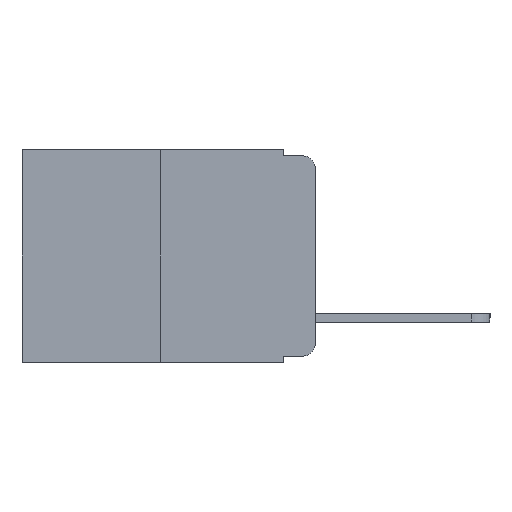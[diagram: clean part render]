
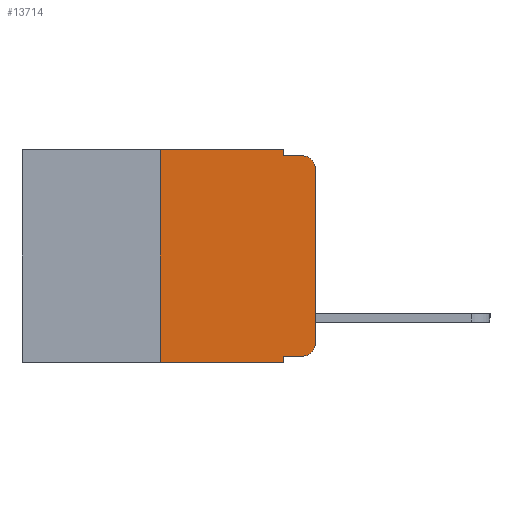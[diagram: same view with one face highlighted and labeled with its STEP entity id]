
A CAD part, left-side view. The second image highlights one B-rep face of the part: STEP entity #13714.
In plain terms, the highlighted planar face has unit normal (-1, 0, 0).
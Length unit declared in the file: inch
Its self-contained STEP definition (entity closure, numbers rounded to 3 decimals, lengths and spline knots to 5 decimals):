
#218 = VECTOR ( 'NONE', #4773, 39.37008 ) ;
#249 = AXIS2_PLACEMENT_3D ( 'NONE', #5105, #11500, #5154 ) ;
#748 = LINE ( 'NONE', #1525, #9641 ) ;
#808 = CARTESIAN_POINT ( 'NONE',  ( 0., 0.25, 0. ) ) ;
#854 = EDGE_CURVE ( 'NONE', #11794, #7351, #8269, .T. ) ;
#1036 = EDGE_CURVE ( 'NONE', #11684, #6754, #11219, .T. ) ;
#1085 = DIRECTION ( 'NONE',  ( -1., 0., 0. ) ) ;
#1188 = CARTESIAN_POINT ( 'NONE',  ( 0., 0.02, -0.333 ) ) ;
#1525 = CARTESIAN_POINT ( 'NONE',  ( 0., 0.473, 0. ) ) ;
#1909 = PLANE ( 'NONE',  #249 ) ;
#2154 = CIRCLE ( 'NONE', #10046, 0.02 ) ;
#2180 = ORIENTED_EDGE ( 'NONE', *, *, #4214, .F. ) ;
#2294 = CARTESIAN_POINT ( 'NONE',  ( 0., 0.051, -0.01 ) ) ;
#2528 = EDGE_CURVE ( 'NONE', #7351, #7688, #5343, .T. ) ;
#2683 = CARTESIAN_POINT ( 'NONE',  ( 0., 0., -0.313 ) ) ;
#3416 = CARTESIAN_POINT ( 'NONE',  ( 0., 0.051, -0.01 ) ) ;
#3449 = CARTESIAN_POINT ( 'NONE',  ( 0., 0.051, -0.343 ) ) ;
#3455 = EDGE_CURVE ( 'NONE', #4340, #9997, #6809, .T. ) ;
#3601 = CARTESIAN_POINT ( 'NONE',  ( 0., 0.02, -0.313 ) ) ;
#3839 = ORIENTED_EDGE ( 'NONE', *, *, #2528, .T. ) ;
#4214 = EDGE_CURVE ( 'NONE', #6754, #10799, #748, .T. ) ;
#4245 = EDGE_CURVE ( 'NONE', #11835, #6197, #5792, .T. ) ;
#4275 = VECTOR ( 'NONE', #12640, 39.37008 ) ;
#4340 = VERTEX_POINT ( 'NONE', #12952 ) ;
#4430 = DIRECTION ( 'NONE',  ( 0., -1., 0. ) ) ;
#4698 = ORIENTED_EDGE ( 'NONE', *, *, #5234, .F. ) ;
#4773 = DIRECTION ( 'NONE',  ( 0., 0., 1. ) ) ;
#4866 = ORIENTED_EDGE ( 'NONE', *, *, #9236, .T. ) ;
#5105 = CARTESIAN_POINT ( 'NONE',  ( 0., 0.473, 0. ) ) ;
#5154 = DIRECTION ( 'NONE',  ( 0., 0., -1. ) ) ;
#5234 = EDGE_CURVE ( 'NONE', #10799, #11835, #7107, .T. ) ;
#5343 = LINE ( 'NONE', #9181, #10650 ) ;
#5631 = VECTOR ( 'NONE', #13531, 39.37008 ) ;
#5707 = CARTESIAN_POINT ( 'NONE',  ( 0., 0.051, 0. ) ) ;
#5792 = LINE ( 'NONE', #2294, #11431 ) ;
#5940 = LINE ( 'NONE', #13579, #11244 ) ;
#6018 = ORIENTED_EDGE ( 'NONE', *, *, #6727, .T. ) ;
#6197 = VERTEX_POINT ( 'NONE', #6860 ) ;
#6575 = DIRECTION ( 'NONE',  ( 0., -1., 0. ) ) ;
#6727 = EDGE_CURVE ( 'NONE', #11684, #9997, #11610, .T. ) ;
#6754 = VERTEX_POINT ( 'NONE', #808 ) ;
#6809 = LINE ( 'NONE', #11252, #9307 ) ;
#6849 = DIRECTION ( 'NONE',  ( -1., 0., 0. ) ) ;
#6860 = CARTESIAN_POINT ( 'NONE',  ( 0., 0.02, -0.01 ) ) ;
#7107 = LINE ( 'NONE', #5707, #4275 ) ;
#7212 = DIRECTION ( 'NONE',  ( 0., 0., -1. ) ) ;
#7351 = VERTEX_POINT ( 'NONE', #2683 ) ;
#7504 = CARTESIAN_POINT ( 'NONE',  ( 0., 0.02, -0.03 ) ) ;
#7688 = VERTEX_POINT ( 'NONE', #13433 ) ;
#7718 = CARTESIAN_POINT ( 'NONE',  ( 0., 0.25, 0. ) ) ;
#8189 = DIRECTION ( 'NONE',  ( 0., 0., -1. ) ) ;
#8269 = CIRCLE ( 'NONE', #8898, 0.02 ) ;
#8362 = DIRECTION ( 'NONE',  ( 0., -1., 0. ) ) ;
#8593 = DIRECTION ( 'NONE',  ( 0., 0., -1. ) ) ;
#8898 = AXIS2_PLACEMENT_3D ( 'NONE', #3601, #6849, #7212 ) ;
#9177 = DIRECTION ( 'NONE',  ( 0., 0., 1. ) ) ;
#9181 = CARTESIAN_POINT ( 'NONE',  ( 0., 0., 0. ) ) ;
#9236 = EDGE_CURVE ( 'NONE', #7688, #6197, #2154, .T. ) ;
#9241 = EDGE_LOOP ( 'NONE', ( #3839, #4866, #11827, #4698, #2180, #11332, #6018, #9847, #13621, #12162 ) ) ;
#9307 = VECTOR ( 'NONE', #8189, 39.37008 ) ;
#9485 = CARTESIAN_POINT ( 'NONE',  ( 0., 0.473, -0.343 ) ) ;
#9641 = VECTOR ( 'NONE', #4430, 39.37008 ) ;
#9847 = ORIENTED_EDGE ( 'NONE', *, *, #3455, .F. ) ;
#9997 = VERTEX_POINT ( 'NONE', #3449 ) ;
#10046 = AXIS2_PLACEMENT_3D ( 'NONE', #7504, #1085, #8593 ) ;
#10650 = VECTOR ( 'NONE', #9177, 39.37008 ) ;
#10799 = VERTEX_POINT ( 'NONE', #11181 ) ;
#11181 = CARTESIAN_POINT ( 'NONE',  ( 0., 0.051, 0. ) ) ;
#11219 = LINE ( 'NONE', #7718, #218 ) ;
#11244 = VECTOR ( 'NONE', #8362, 39.37008 ) ;
#11252 = CARTESIAN_POINT ( 'NONE',  ( 0., 0.051, 0. ) ) ;
#11332 = ORIENTED_EDGE ( 'NONE', *, *, #1036, .F. ) ;
#11431 = VECTOR ( 'NONE', #6575, 39.37008 ) ;
#11500 = DIRECTION ( 'NONE',  ( 1., 0., 0. ) ) ;
#11578 = EDGE_CURVE ( 'NONE', #4340, #11794, #5940, .T. ) ;
#11610 = LINE ( 'NONE', #9485, #5631 ) ;
#11684 = VERTEX_POINT ( 'NONE', #13750 ) ;
#11794 = VERTEX_POINT ( 'NONE', #1188 ) ;
#11827 = ORIENTED_EDGE ( 'NONE', *, *, #4245, .F. ) ;
#11835 = VERTEX_POINT ( 'NONE', #3416 ) ;
#12162 = ORIENTED_EDGE ( 'NONE', *, *, #854, .T. ) ;
#12640 = DIRECTION ( 'NONE',  ( 0., 0., -1. ) ) ;
#12952 = CARTESIAN_POINT ( 'NONE',  ( 0., 0.051, -0.333 ) ) ;
#13318 = FACE_OUTER_BOUND ( 'NONE', #9241, .T. ) ;
#13433 = CARTESIAN_POINT ( 'NONE',  ( 0., 0., -0.03 ) ) ;
#13531 = DIRECTION ( 'NONE',  ( 0., -1., 0. ) ) ;
#13579 = CARTESIAN_POINT ( 'NONE',  ( 0., 0.051, -0.333 ) ) ;
#13621 = ORIENTED_EDGE ( 'NONE', *, *, #11578, .T. ) ;
#13714 = ADVANCED_FACE ( 'NONE', ( #13318 ), #1909, .F. ) ;
#13750 = CARTESIAN_POINT ( 'NONE',  ( 0., 0.25, -0.343 ) ) ;
